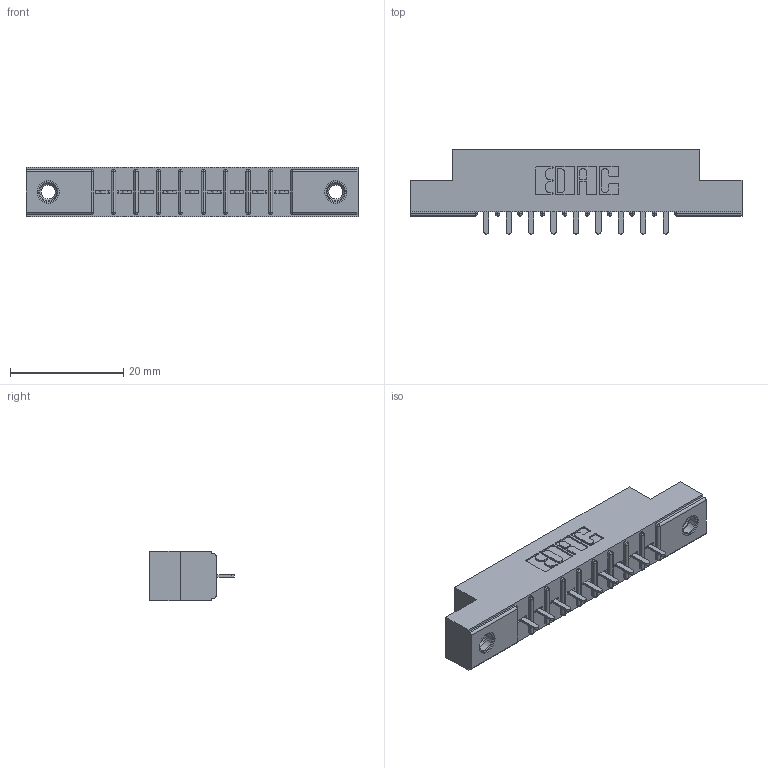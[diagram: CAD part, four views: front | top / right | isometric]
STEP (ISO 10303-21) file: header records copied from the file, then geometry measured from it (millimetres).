
FILE_DESCRIPTION (( 'STEP AP203' ), '1' );
FILE_NAME ('316-009-421-107.STEP', '2020-09-22T15:04:03', ( '' ), ( '' ), 'SwSTEP 2.0', 'SolidWorks 2020', '' );
FILE_SCHEMA (( 'CONFIG_CONTROL_DESIGN' ));
Length unit declared in the file: inch
Products named in the file (4): 345-250-001_345-250-005-103; 316-009-421-107; 306 Part_.156 Dia; 306-290-001_121
Assembly tree (12 placements, depth 2):
  316-009-421-107
    306 Part_.156 Dia
    306-290-001_121  x9
    345-250-001_345-250-005-103  x2
Bounding box: 58.67 x 14.88 x 8.71 mm (x, y, z)
Volume: 3934.4 mm3; surface area: 5374.8 mm2
Topology: 12 solids, 12 shells, 806 faces, 2225 edges, 1426 vertices
Faces by surface type: plane 523, cylinder 231, sphere 36, cone 12, torus 4
Entity records: 13809 total; most frequent: CARTESIAN_POINT 2293, DIRECTION 2273, ORIENTED_EDGE 2262, EDGE_CURVE 1131, VECTOR 865, LINE 865, VERTEX_POINT 724, AXIS2_PLACEMENT_3D 704
